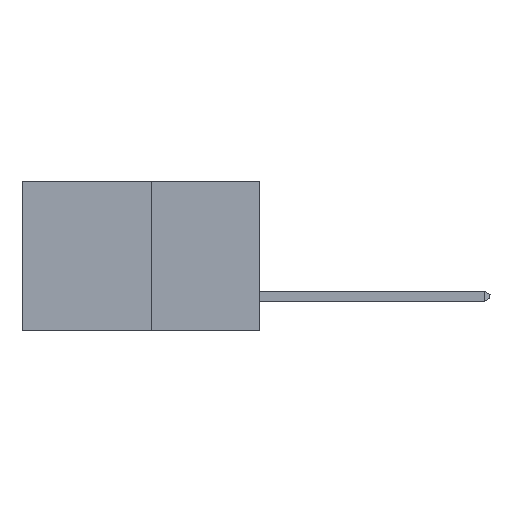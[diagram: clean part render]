
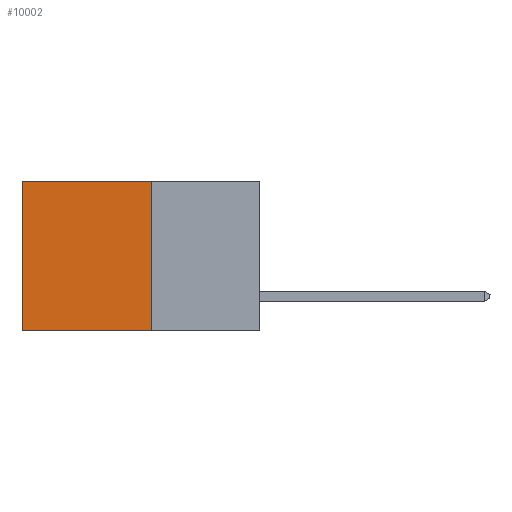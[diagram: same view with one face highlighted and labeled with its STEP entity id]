
A CAD part, left-side view. The second image highlights one B-rep face of the part: STEP entity #10002.
In plain terms, the highlighted planar face has unit normal (-1, 0, 0).
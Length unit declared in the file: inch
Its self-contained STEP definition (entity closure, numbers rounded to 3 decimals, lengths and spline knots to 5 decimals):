
#220 = EDGE_LOOP ( 'NONE', ( #594, #4034, #6750, #10850 ) ) ;
#594 = ORIENTED_EDGE ( 'NONE', *, *, #3482, .T. ) ;
#1105 = DIRECTION ( 'NONE',  ( 0., 1., 0. ) ) ;
#1264 = EDGE_CURVE ( 'NONE', #13435, #3306, #12623, .T. ) ;
#1390 = VECTOR ( 'NONE', #13310, 39.37008 ) ;
#2393 = CARTESIAN_POINT ( 'NONE',  ( 0.277, 0.27, 0. ) ) ;
#2854 = VECTOR ( 'NONE', #2889, 39.37008 ) ;
#2862 = CARTESIAN_POINT ( 'NONE',  ( 0.277, 0.59, -0.37 ) ) ;
#2889 = DIRECTION ( 'NONE',  ( 0., 0., -1. ) ) ;
#3306 = VERTEX_POINT ( 'NONE', #8066 ) ;
#3482 = EDGE_CURVE ( 'NONE', #3306, #10236, #8460, .T. ) ;
#3630 = CARTESIAN_POINT ( 'NONE',  ( 0.277, 0.59, -0.37 ) ) ;
#3676 = LINE ( 'NONE', #13388, #9194 ) ;
#4034 = ORIENTED_EDGE ( 'NONE', *, *, #7891, .F. ) ;
#4298 = CARTESIAN_POINT ( 'NONE',  ( 0.277, 0.27, -0.37 ) ) ;
#4353 = LINE ( 'NONE', #7264, #1390 ) ;
#5363 = DIRECTION ( 'NONE',  ( 1., 0., 0. ) ) ;
#6594 = FACE_OUTER_BOUND ( 'NONE', #220, .T. ) ;
#6750 = ORIENTED_EDGE ( 'NONE', *, *, #7848, .F. ) ;
#7264 = CARTESIAN_POINT ( 'NONE',  ( 0.277, 0.27, -0.37 ) ) ;
#7362 = DIRECTION ( 'NONE',  ( 0., 1., 0. ) ) ;
#7848 = EDGE_CURVE ( 'NONE', #13435, #11040, #4353, .T. ) ;
#7891 = EDGE_CURVE ( 'NONE', #11040, #10236, #3676, .T. ) ;
#8066 = CARTESIAN_POINT ( 'NONE',  ( 0.277, 0.59, 0. ) ) ;
#8129 = CARTESIAN_POINT ( 'NONE',  ( 0.277, 0.27, -0.37 ) ) ;
#8460 = LINE ( 'NONE', #2862, #2854 ) ;
#9194 = VECTOR ( 'NONE', #7362, 39.37008 ) ;
#9911 = VECTOR ( 'NONE', #1105, 39.37008 ) ;
#10002 = ADVANCED_FACE ( 'NONE', ( #6594 ), #10453, .F. ) ;
#10172 = CARTESIAN_POINT ( 'NONE',  ( 0.277, 0.27, 0. ) ) ;
#10236 = VERTEX_POINT ( 'NONE', #3630 ) ;
#10453 = PLANE ( 'NONE',  #10806 ) ;
#10806 = AXIS2_PLACEMENT_3D ( 'NONE', #4298, #5363, #12500 ) ;
#10850 = ORIENTED_EDGE ( 'NONE', *, *, #1264, .T. ) ;
#11040 = VERTEX_POINT ( 'NONE', #8129 ) ;
#12500 = DIRECTION ( 'NONE',  ( 0., 0., -1. ) ) ;
#12623 = LINE ( 'NONE', #2393, #9911 ) ;
#13310 = DIRECTION ( 'NONE',  ( 0., 0., -1. ) ) ;
#13388 = CARTESIAN_POINT ( 'NONE',  ( 0.277, 0.27, -0.37 ) ) ;
#13435 = VERTEX_POINT ( 'NONE', #10172 ) ;
